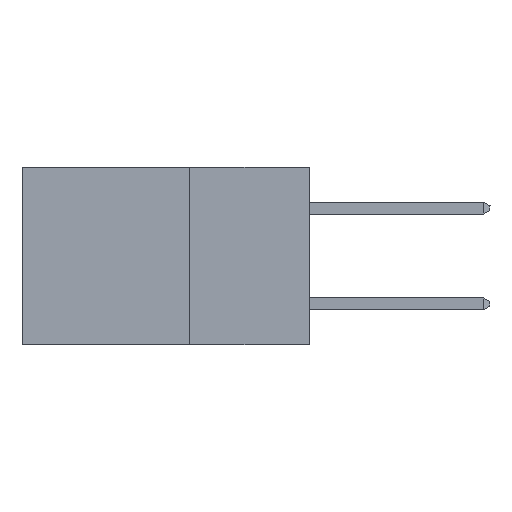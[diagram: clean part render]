
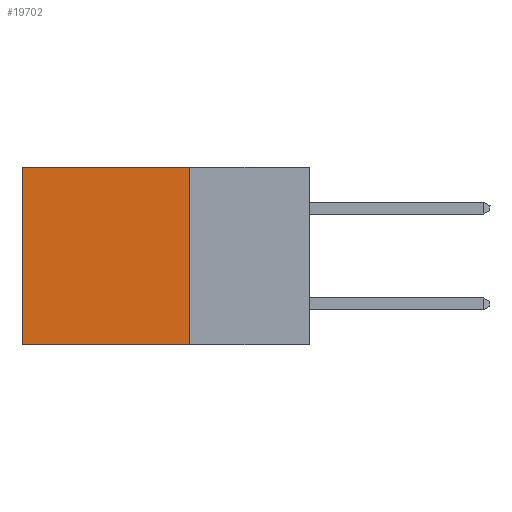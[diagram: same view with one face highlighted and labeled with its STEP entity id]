
A CAD part, left-side view. The second image highlights one B-rep face of the part: STEP entity #19702.
In plain terms, the highlighted planar face has unit normal (-1, 0, 0).
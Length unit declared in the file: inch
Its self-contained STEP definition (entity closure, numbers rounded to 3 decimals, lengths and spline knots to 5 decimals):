
#656 = VERTEX_POINT ( 'NONE', #19274 ) ;
#1124 = EDGE_CURVE ( 'NONE', #4747, #1665, #18831, .T. ) ;
#1368 = EDGE_CURVE ( 'NONE', #1665, #656, #1748, .T. ) ;
#1665 = VERTEX_POINT ( 'NONE', #2826 ) ;
#1748 = LINE ( 'NONE', #27413, #17148 ) ;
#1781 = CARTESIAN_POINT ( 'NONE',  ( 0.2875, 0.25, 0. ) ) ;
#2757 = PLANE ( 'NONE',  #6063 ) ;
#2826 = CARTESIAN_POINT ( 'NONE',  ( 0.2875, 0.25, -0.37 ) ) ;
#4747 = VERTEX_POINT ( 'NONE', #8000 ) ;
#4975 = ORIENTED_EDGE ( 'NONE', *, *, #18688, .T. ) ;
#5168 = VECTOR ( 'NONE', #17093, 39.37008 ) ;
#5608 = EDGE_CURVE ( 'NONE', #4747, #20894, #14184, .T. ) ;
#6063 = AXIS2_PLACEMENT_3D ( 'NONE', #11256, #22156, #16426 ) ;
#6554 = VECTOR ( 'NONE', #27310, 39.37008 ) ;
#7481 = ORIENTED_EDGE ( 'NONE', *, *, #1124, .F. ) ;
#8000 = CARTESIAN_POINT ( 'NONE',  ( 0.2875, 0.25, 0. ) ) ;
#8594 = CARTESIAN_POINT ( 'NONE',  ( 0.2875, 0.6, 0. ) ) ;
#9886 = EDGE_LOOP ( 'NONE', ( #4975, #16793, #7481, #17522 ) ) ;
#11256 = CARTESIAN_POINT ( 'NONE',  ( 0.2875, 0.25, 0. ) ) ;
#12197 = DIRECTION ( 'NONE',  ( 0., 1., 0. ) ) ;
#13086 = CARTESIAN_POINT ( 'NONE',  ( 0.2875, 0.25, 0. ) ) ;
#14184 = LINE ( 'NONE', #1781, #6554 ) ;
#16426 = DIRECTION ( 'NONE',  ( 0., 0., -1. ) ) ;
#16793 = ORIENTED_EDGE ( 'NONE', *, *, #1368, .F. ) ;
#16962 = LINE ( 'NONE', #8594, #5168 ) ;
#17093 = DIRECTION ( 'NONE',  ( 0., 0., -1. ) ) ;
#17142 = DIRECTION ( 'NONE',  ( 0., 0., -1. ) ) ;
#17148 = VECTOR ( 'NONE', #12197, 39.37008 ) ;
#17522 = ORIENTED_EDGE ( 'NONE', *, *, #5608, .T. ) ;
#18688 = EDGE_CURVE ( 'NONE', #20894, #656, #16962, .T. ) ;
#18831 = LINE ( 'NONE', #13086, #26075 ) ;
#19274 = CARTESIAN_POINT ( 'NONE',  ( 0.2875, 0.6, -0.37 ) ) ;
#19702 = ADVANCED_FACE ( 'NONE', ( #21879 ), #2757, .F. ) ;
#20894 = VERTEX_POINT ( 'NONE', #24378 ) ;
#21879 = FACE_OUTER_BOUND ( 'NONE', #9886, .T. ) ;
#22156 = DIRECTION ( 'NONE',  ( 1., 0., 0. ) ) ;
#24378 = CARTESIAN_POINT ( 'NONE',  ( 0.2875, 0.6, 0. ) ) ;
#26075 = VECTOR ( 'NONE', #17142, 39.37008 ) ;
#27310 = DIRECTION ( 'NONE',  ( 0., 1., 0. ) ) ;
#27413 = CARTESIAN_POINT ( 'NONE',  ( 0.2875, 0.25, -0.37 ) ) ;
